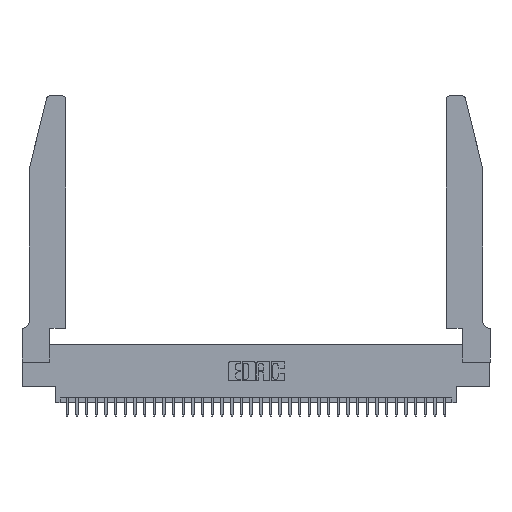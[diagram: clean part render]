
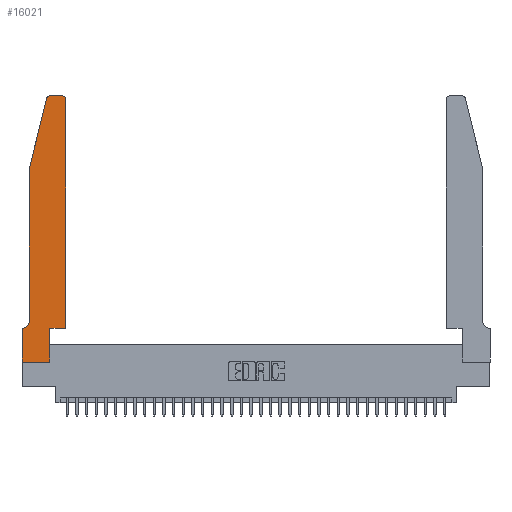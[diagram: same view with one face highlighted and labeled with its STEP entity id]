
A CAD part, top view. The second image highlights one B-rep face of the part: STEP entity #16021.
In plain terms, the highlighted planar face has unit normal (0, 0, 1).
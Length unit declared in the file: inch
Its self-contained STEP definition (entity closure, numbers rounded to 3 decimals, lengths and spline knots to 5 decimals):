
#806 = CARTESIAN_POINT ( 'NONE',  ( 0.4505, 0.35, 0.37 ) ) ;
#1461 = ORIENTED_EDGE ( 'NONE', *, *, #10512, .T. ) ;
#1465 = DIRECTION ( 'NONE',  ( 0., 0., 1. ) ) ;
#2197 = VECTOR ( 'NONE', #4296, 39.37008 ) ;
#2347 = CARTESIAN_POINT ( 'NONE',  ( 0.2865, 0., 0.37 ) ) ;
#2625 = VERTEX_POINT ( 'NONE', #27081 ) ;
#2649 = DIRECTION ( 'NONE',  ( 0., 1., 0. ) ) ;
#2784 = LINE ( 'NONE', #18272, #13370 ) ;
#2919 = VECTOR ( 'NONE', #4779, 39.37008 ) ;
#3652 = ORIENTED_EDGE ( 'NONE', *, *, #32106, .T. ) ;
#3942 = EDGE_CURVE ( 'NONE', #4397, #23850, #22517, .T. ) ;
#4296 = DIRECTION ( 'NONE',  ( 0., -1., 0. ) ) ;
#4397 = VERTEX_POINT ( 'NONE', #28154 ) ;
#4423 = DIRECTION ( 'NONE',  ( 0., 0., -1. ) ) ;
#4779 = DIRECTION ( 'NONE',  ( 0., -1., 0. ) ) ;
#5443 = VECTOR ( 'NONE', #2649, 39.37008 ) ;
#5474 = EDGE_CURVE ( 'NONE', #2625, #11981, #21052, .T. ) ;
#5488 = VECTOR ( 'NONE', #33090, 39.37008 ) ;
#5898 = CARTESIAN_POINT ( 'NONE',  ( 0., 0.35, 0.37 ) ) ;
#6351 = EDGE_CURVE ( 'NONE', #23850, #2625, #14081, .T. ) ;
#6853 = CARTESIAN_POINT ( 'NONE',  ( 0.0755, 2., 0.37 ) ) ;
#7328 = CARTESIAN_POINT ( 'NONE',  ( 0.25487, 2.72718, 0.37 ) ) ;
#7555 = CARTESIAN_POINT ( 'NONE',  ( 0.2865, 0.35, 0.37 ) ) ;
#7979 = VERTEX_POINT ( 'NONE', #36189 ) ;
#8872 = CARTESIAN_POINT ( 'NONE',  ( 0., 0., 0.37 ) ) ;
#8877 = DIRECTION ( 'NONE',  ( 0., 0., 1. ) ) ;
#9263 = VERTEX_POINT ( 'NONE', #21811 ) ;
#9472 = EDGE_CURVE ( 'NONE', #17731, #21045, #17427, .T. ) ;
#10512 = EDGE_CURVE ( 'NONE', #28080, #20116, #23977, .T. ) ;
#10563 = CARTESIAN_POINT ( 'NONE',  ( 0.4505, 0.35, 0.37 ) ) ;
#11118 = EDGE_CURVE ( 'NONE', #35040, #17731, #2784, .T. ) ;
#11981 = VERTEX_POINT ( 'NONE', #7328 ) ;
#12492 = DIRECTION ( 'NONE',  ( 1., 0., 0. ) ) ;
#12553 = CIRCLE ( 'NONE', #25335, 0.07 ) ;
#12884 = CARTESIAN_POINT ( 'NONE',  ( 0., 0., 0.37 ) ) ;
#12945 = ORIENTED_EDGE ( 'NONE', *, *, #11118, .T. ) ;
#13370 = VECTOR ( 'NONE', #15809, 39.37008 ) ;
#13649 = CARTESIAN_POINT ( 'NONE',  ( 0.4205, 2.75, 0.37 ) ) ;
#14081 = LINE ( 'NONE', #19927, #20670 ) ;
#14302 = DIRECTION ( 'NONE',  ( 1., 0., 0. ) ) ;
#14839 = ORIENTED_EDGE ( 'NONE', *, *, #22593, .T. ) ;
#15259 = EDGE_CURVE ( 'NONE', #11981, #7979, #15717, .T. ) ;
#15708 = PLANE ( 'NONE',  #18829 ) ;
#15717 = LINE ( 'NONE', #19366, #22838 ) ;
#15809 = DIRECTION ( 'NONE',  ( -1., 0., 0. ) ) ;
#15885 = CARTESIAN_POINT ( 'NONE',  ( 0., 0., 0.37 ) ) ;
#16021 = ADVANCED_FACE ( 'NONE', ( #24062 ), #15708, .T. ) ;
#16092 = CARTESIAN_POINT ( 'NONE',  ( 0.4505, 0.35, 0.37 ) ) ;
#17230 = EDGE_CURVE ( 'NONE', #20116, #22759, #19207, .T. ) ;
#17249 = ORIENTED_EDGE ( 'NONE', *, *, #3942, .T. ) ;
#17427 = LINE ( 'NONE', #8872, #2919 ) ;
#17539 = CARTESIAN_POINT ( 'NONE',  ( 0.0055, 0.35, 0.37 ) ) ;
#17731 = VERTEX_POINT ( 'NONE', #5898 ) ;
#17959 = DIRECTION ( 'NONE',  ( 1., 0., 0. ) ) ;
#18272 = CARTESIAN_POINT ( 'NONE',  ( 0.0755, 0.35, 0.37 ) ) ;
#18829 = AXIS2_PLACEMENT_3D ( 'NONE', #34932, #1465, #12492 ) ;
#19207 = LINE ( 'NONE', #10563, #5488 ) ;
#19288 = AXIS2_PLACEMENT_3D ( 'NONE', #25570, #8877, #17959 ) ;
#19366 = CARTESIAN_POINT ( 'NONE',  ( 0.0755, 2., 0.37 ) ) ;
#19496 = DIRECTION ( 'NONE',  ( -0.239, -0.971, 0. ) ) ;
#19927 = CARTESIAN_POINT ( 'NONE',  ( 0.2605, 2.75, 0.37 ) ) ;
#20116 = VERTEX_POINT ( 'NONE', #26478 ) ;
#20670 = VECTOR ( 'NONE', #36132, 39.37008 ) ;
#21045 = VERTEX_POINT ( 'NONE', #12884 ) ;
#21052 = CIRCLE ( 'NONE', #34569, 0.03 ) ;
#21068 = LINE ( 'NONE', #806, #27730 ) ;
#21719 = EDGE_CURVE ( 'NONE', #22759, #4397, #21068, .T. ) ;
#21724 = DIRECTION ( 'NONE',  ( 1., 0., 0. ) ) ;
#21811 = CARTESIAN_POINT ( 'NONE',  ( 0.0755, 0.42, 0.37 ) ) ;
#22365 = VECTOR ( 'NONE', #21724, 39.37008 ) ;
#22517 = CIRCLE ( 'NONE', #19288, 0.03 ) ;
#22593 = EDGE_CURVE ( 'NONE', #21045, #28080, #24571, .T. ) ;
#22759 = VERTEX_POINT ( 'NONE', #16092 ) ;
#22838 = VECTOR ( 'NONE', #19496, 39.37008 ) ;
#23542 = ORIENTED_EDGE ( 'NONE', *, *, #21719, .T. ) ;
#23802 = LINE ( 'NONE', #6853, #2197 ) ;
#23850 = VERTEX_POINT ( 'NONE', #13649 ) ;
#23977 = LINE ( 'NONE', #7555, #5443 ) ;
#24062 = FACE_OUTER_BOUND ( 'NONE', #28525, .T. ) ;
#24229 = ORIENTED_EDGE ( 'NONE', *, *, #17230, .T. ) ;
#24571 = LINE ( 'NONE', #15885, #22365 ) ;
#25335 = AXIS2_PLACEMENT_3D ( 'NONE', #35373, #4423, #26996 ) ;
#25570 = CARTESIAN_POINT ( 'NONE',  ( 0.4205, 2.72, 0.37 ) ) ;
#26478 = CARTESIAN_POINT ( 'NONE',  ( 0.2865, 0.35, 0.37 ) ) ;
#26996 = DIRECTION ( 'NONE',  ( -1., 0., 0. ) ) ;
#27081 = CARTESIAN_POINT ( 'NONE',  ( 0.284, 2.75, 0.37 ) ) ;
#27187 = ORIENTED_EDGE ( 'NONE', *, *, #6351, .T. ) ;
#27730 = VECTOR ( 'NONE', #29225, 39.37008 ) ;
#28016 = CARTESIAN_POINT ( 'NONE',  ( 0.284, 2.72, 0.37 ) ) ;
#28080 = VERTEX_POINT ( 'NONE', #2347 ) ;
#28154 = CARTESIAN_POINT ( 'NONE',  ( 0.4505, 2.72, 0.37 ) ) ;
#28295 = ORIENTED_EDGE ( 'NONE', *, *, #9472, .T. ) ;
#28525 = EDGE_LOOP ( 'NONE', ( #27187, #31745, #35870, #3652, #33748, #12945, #28295, #14839, #1461, #24229, #23542, #17249 ) ) ;
#29080 = EDGE_CURVE ( 'NONE', #9263, #35040, #12553, .T. ) ;
#29225 = DIRECTION ( 'NONE',  ( 0., 1., 0. ) ) ;
#31745 = ORIENTED_EDGE ( 'NONE', *, *, #5474, .T. ) ;
#32106 = EDGE_CURVE ( 'NONE', #7979, #9263, #23802, .T. ) ;
#33090 = DIRECTION ( 'NONE',  ( 1., 0., 0. ) ) ;
#33652 = DIRECTION ( 'NONE',  ( 0., 0., 1. ) ) ;
#33748 = ORIENTED_EDGE ( 'NONE', *, *, #29080, .T. ) ;
#34569 = AXIS2_PLACEMENT_3D ( 'NONE', #28016, #33652, #14302 ) ;
#34932 = CARTESIAN_POINT ( 'NONE',  ( 0., 0.35, 0.37 ) ) ;
#35040 = VERTEX_POINT ( 'NONE', #17539 ) ;
#35373 = CARTESIAN_POINT ( 'NONE',  ( 0.0055, 0.42, 0.37 ) ) ;
#35870 = ORIENTED_EDGE ( 'NONE', *, *, #15259, .T. ) ;
#36132 = DIRECTION ( 'NONE',  ( -1., 0., 0. ) ) ;
#36189 = CARTESIAN_POINT ( 'NONE',  ( 0.0755, 2., 0.37 ) ) ;
